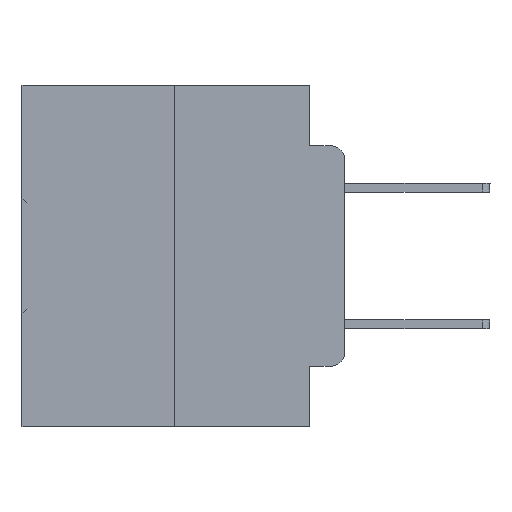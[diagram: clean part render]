
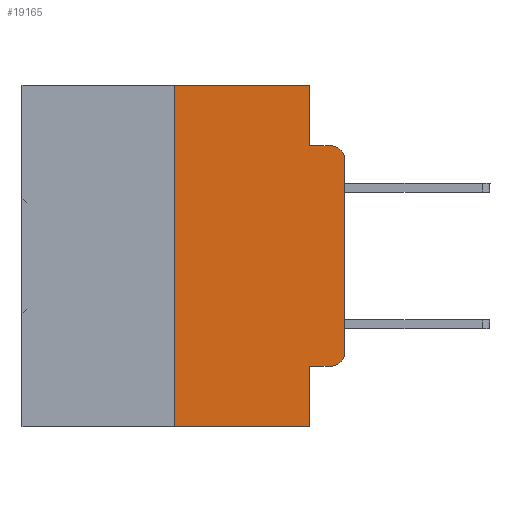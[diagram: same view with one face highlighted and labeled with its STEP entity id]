
A CAD part, left-side view. The second image highlights one B-rep face of the part: STEP entity #19165.
In plain terms, the highlighted planar face has unit normal (-1, 0, 0).
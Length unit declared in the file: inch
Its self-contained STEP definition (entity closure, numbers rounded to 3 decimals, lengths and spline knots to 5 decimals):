
#168 = CARTESIAN_POINT ( 'NONE',  ( 0., 0.051, -0.4115 ) ) ;
#268 = EDGE_CURVE ( 'NONE', #13921, #21338, #27857, .T. ) ;
#287 = DIRECTION ( 'NONE',  ( 0., 0., -1. ) ) ;
#2531 = VERTEX_POINT ( 'NONE', #30702 ) ;
#2684 = AXIS2_PLACEMENT_3D ( 'NONE', #8444, #6106, #8863 ) ;
#2769 = VECTOR ( 'NONE', #20705, 39.37008 ) ;
#2892 = EDGE_CURVE ( 'NONE', #21338, #19486, #15904, .T. ) ;
#3766 = CARTESIAN_POINT ( 'NONE',  ( 0., 0.051, 0. ) ) ;
#4029 = DIRECTION ( 'NONE',  ( 0., 0., 1. ) ) ;
#4135 = VECTOR ( 'NONE', #287, 39.37008 ) ;
#5110 = VECTOR ( 'NONE', #7338, 39.37008 ) ;
#5407 = EDGE_LOOP ( 'NONE', ( #19852, #27312, #27087, #22380, #25890, #24541, #22923, #19632, #21992, #17301 ) ) ;
#5766 = CARTESIAN_POINT ( 'NONE',  ( 0., 0.25, 0. ) ) ;
#6082 = CIRCLE ( 'NONE', #2684, 0.02 ) ;
#6106 = DIRECTION ( 'NONE',  ( -1., 0., 0. ) ) ;
#6263 = VERTEX_POINT ( 'NONE', #30501 ) ;
#6572 = PLANE ( 'NONE',  #32236 ) ;
#7150 = VERTEX_POINT ( 'NONE', #5766 ) ;
#7338 = DIRECTION ( 'NONE',  ( 0., -1., 0. ) ) ;
#8012 = VECTOR ( 'NONE', #13457, 39.37008 ) ;
#8444 = CARTESIAN_POINT ( 'NONE',  ( 0., 0.02, -0.1085 ) ) ;
#8691 = CARTESIAN_POINT ( 'NONE',  ( 0., 0.473, 0. ) ) ;
#8863 = DIRECTION ( 'NONE',  ( 0., 0., -1. ) ) ;
#9545 = VECTOR ( 'NONE', #21450, 39.37008 ) ;
#10773 = EDGE_CURVE ( 'NONE', #2531, #11921, #25281, .T. ) ;
#10926 = EDGE_CURVE ( 'NONE', #6263, #7150, #30039, .T. ) ;
#11033 = VERTEX_POINT ( 'NONE', #28627 ) ;
#11881 = EDGE_CURVE ( 'NONE', #11921, #11033, #27596, .T. ) ;
#11921 = VERTEX_POINT ( 'NONE', #22830 ) ;
#11940 = LINE ( 'NONE', #3766, #9545 ) ;
#12979 = LINE ( 'NONE', #20556, #16529 ) ;
#13003 = DIRECTION ( 'NONE',  ( -1., 0., 0. ) ) ;
#13457 = DIRECTION ( 'NONE',  ( 0., -1., 0. ) ) ;
#13702 = CARTESIAN_POINT ( 'NONE',  ( 0., 0., -0.1085 ) ) ;
#13921 = VERTEX_POINT ( 'NONE', #21578 ) ;
#15428 = LINE ( 'NONE', #30982, #2769 ) ;
#15442 = DIRECTION ( 'NONE',  ( 0., 0., -1. ) ) ;
#15904 = LINE ( 'NONE', #20956, #8012 ) ;
#16055 = CARTESIAN_POINT ( 'NONE',  ( 0., 0.051, -0.5 ) ) ;
#16215 = DIRECTION ( 'NONE',  ( 0., 0., -1. ) ) ;
#16225 = EDGE_CURVE ( 'NONE', #2531, #22516, #11940, .T. ) ;
#16529 = VECTOR ( 'NONE', #28057, 39.37008 ) ;
#16648 = CARTESIAN_POINT ( 'NONE',  ( 0., 0., 0. ) ) ;
#16725 = VECTOR ( 'NONE', #4029, 39.37008 ) ;
#17301 = ORIENTED_EDGE ( 'NONE', *, *, #11881, .T. ) ;
#17637 = CARTESIAN_POINT ( 'NONE',  ( 0., 0.02, -0.0885 ) ) ;
#17983 = CARTESIAN_POINT ( 'NONE',  ( 0., 0.02, -0.3915 ) ) ;
#18374 = CARTESIAN_POINT ( 'NONE',  ( 0., 0.25, 0. ) ) ;
#19165 = ADVANCED_FACE ( 'NONE', ( #27003 ), #6572, .F. ) ;
#19267 = EDGE_CURVE ( 'NONE', #11033, #31055, #31740, .T. ) ;
#19486 = VERTEX_POINT ( 'NONE', #17637 ) ;
#19632 = ORIENTED_EDGE ( 'NONE', *, *, #16225, .F. ) ;
#19852 = ORIENTED_EDGE ( 'NONE', *, *, #19267, .T. ) ;
#19952 = CARTESIAN_POINT ( 'NONE',  ( 0., 0.051, -0.0885 ) ) ;
#20556 = CARTESIAN_POINT ( 'NONE',  ( 0., 0.473, -0.5 ) ) ;
#20705 = DIRECTION ( 'NONE',  ( 0., -1., 0. ) ) ;
#20956 = CARTESIAN_POINT ( 'NONE',  ( 0., 0.051, -0.0885 ) ) ;
#21338 = VERTEX_POINT ( 'NONE', #19952 ) ;
#21450 = DIRECTION ( 'NONE',  ( 0., 0., -1. ) ) ;
#21576 = EDGE_CURVE ( 'NONE', #7150, #13921, #15428, .T. ) ;
#21578 = CARTESIAN_POINT ( 'NONE',  ( 0., 0.051, 0. ) ) ;
#21598 = DIRECTION ( 'NONE',  ( 1., 0., 0. ) ) ;
#21992 = ORIENTED_EDGE ( 'NONE', *, *, #10773, .T. ) ;
#22380 = ORIENTED_EDGE ( 'NONE', *, *, #268, .F. ) ;
#22514 = VECTOR ( 'NONE', #30740, 39.37008 ) ;
#22516 = VERTEX_POINT ( 'NONE', #16055 ) ;
#22830 = CARTESIAN_POINT ( 'NONE',  ( 0., 0.02, -0.4115 ) ) ;
#22923 = ORIENTED_EDGE ( 'NONE', *, *, #28789, .T. ) ;
#24541 = ORIENTED_EDGE ( 'NONE', *, *, #10926, .F. ) ;
#25281 = LINE ( 'NONE', #168, #5110 ) ;
#25890 = ORIENTED_EDGE ( 'NONE', *, *, #21576, .F. ) ;
#27003 = FACE_OUTER_BOUND ( 'NONE', #5407, .T. ) ;
#27087 = ORIENTED_EDGE ( 'NONE', *, *, #2892, .F. ) ;
#27312 = ORIENTED_EDGE ( 'NONE', *, *, #30246, .T. ) ;
#27596 = CIRCLE ( 'NONE', #29526, 0.02 ) ;
#27857 = LINE ( 'NONE', #27974, #4135 ) ;
#27974 = CARTESIAN_POINT ( 'NONE',  ( 0., 0.051, 0. ) ) ;
#28057 = DIRECTION ( 'NONE',  ( 0., -1., 0. ) ) ;
#28627 = CARTESIAN_POINT ( 'NONE',  ( 0., 0., -0.3915 ) ) ;
#28789 = EDGE_CURVE ( 'NONE', #6263, #22516, #12979, .T. ) ;
#29526 = AXIS2_PLACEMENT_3D ( 'NONE', #17983, #13003, #15442 ) ;
#30039 = LINE ( 'NONE', #18374, #22514 ) ;
#30246 = EDGE_CURVE ( 'NONE', #31055, #19486, #6082, .T. ) ;
#30501 = CARTESIAN_POINT ( 'NONE',  ( 0., 0.25, -0.5 ) ) ;
#30702 = CARTESIAN_POINT ( 'NONE',  ( 0., 0.051, -0.4115 ) ) ;
#30740 = DIRECTION ( 'NONE',  ( 0., 0., 1. ) ) ;
#30982 = CARTESIAN_POINT ( 'NONE',  ( 0., 0.473, 0. ) ) ;
#31055 = VERTEX_POINT ( 'NONE', #13702 ) ;
#31740 = LINE ( 'NONE', #16648, #16725 ) ;
#32236 = AXIS2_PLACEMENT_3D ( 'NONE', #8691, #21598, #16215 ) ;
